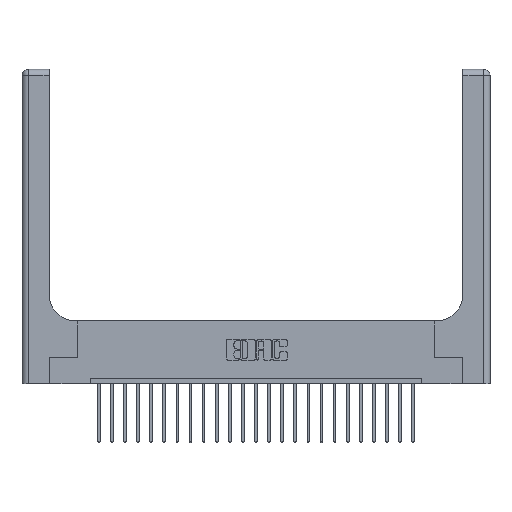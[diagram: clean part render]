
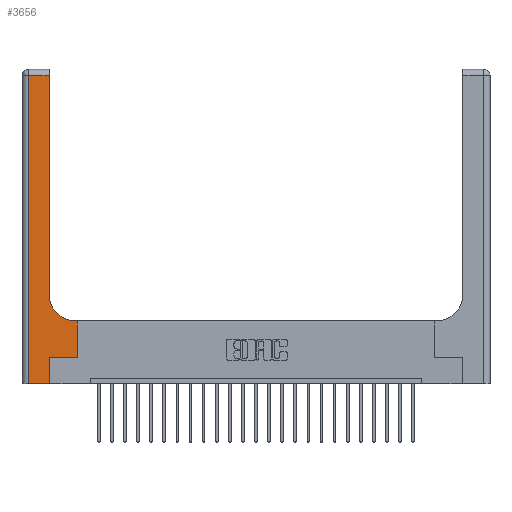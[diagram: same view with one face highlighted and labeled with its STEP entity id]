
A CAD part, top view. The second image highlights one B-rep face of the part: STEP entity #3656.
In plain terms, the highlighted planar face has unit normal (0, 0, 1).
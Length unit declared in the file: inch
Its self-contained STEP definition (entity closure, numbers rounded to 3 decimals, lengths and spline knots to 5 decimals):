
#551 = DIRECTION ( 'NONE',  ( 0., 0., -1. ) ) ;
#799 = VERTEX_POINT ( 'NONE', #23151 ) ;
#1366 = DIRECTION ( 'NONE',  ( 1., 0., 0. ) ) ;
#1512 = ORIENTED_EDGE ( 'NONE', *, *, #6271, .T. ) ;
#1781 = VERTEX_POINT ( 'NONE', #10018 ) ;
#2086 = CARTESIAN_POINT ( 'NONE',  ( 0., 3., 0.37 ) ) ;
#2209 = VECTOR ( 'NONE', #18904, 39.37008 ) ;
#2478 = DIRECTION ( 'NONE',  ( 0., 1., 0. ) ) ;
#2650 = DIRECTION ( 'NONE',  ( 0., 1., 0. ) ) ;
#2822 = CARTESIAN_POINT ( 'NONE',  ( 0.26, 3., 0.37 ) ) ;
#3233 = CARTESIAN_POINT ( 'NONE',  ( 0.528, 0.6, 0.37 ) ) ;
#3656 = ADVANCED_FACE ( 'NONE', ( #11100 ), #14774, .F. ) ;
#3767 = CARTESIAN_POINT ( 'NONE',  ( 0.51, 0.85, 0.37 ) ) ;
#4156 = EDGE_CURVE ( 'NONE', #10062, #5469, #22699, .T. ) ;
#4219 = ORIENTED_EDGE ( 'NONE', *, *, #8851, .T. ) ;
#4439 = CARTESIAN_POINT ( 'NONE',  ( 0.265, 0.25, 0.37 ) ) ;
#5050 = ORIENTED_EDGE ( 'NONE', *, *, #18211, .T. ) ;
#5339 = VECTOR ( 'NONE', #12613, 39.37008 ) ;
#5413 = DIRECTION ( 'NONE',  ( -1., 0., 0. ) ) ;
#5451 = DIRECTION ( 'NONE',  ( 0., 1., 0. ) ) ;
#5469 = VERTEX_POINT ( 'NONE', #4439 ) ;
#5524 = VERTEX_POINT ( 'NONE', #3233 ) ;
#5672 = DIRECTION ( 'NONE',  ( 1., 0., 0. ) ) ;
#6131 = ORIENTED_EDGE ( 'NONE', *, *, #11835, .T. ) ;
#6271 = EDGE_CURVE ( 'NONE', #17594, #15532, #16830, .T. ) ;
#7461 = LINE ( 'NONE', #18607, #12058 ) ;
#7475 = LINE ( 'NONE', #21704, #16451 ) ;
#7657 = ORIENTED_EDGE ( 'NONE', *, *, #4156, .T. ) ;
#7748 = VECTOR ( 'NONE', #2650, 39.37008 ) ;
#7778 = EDGE_CURVE ( 'NONE', #5469, #799, #18783, .T. ) ;
#8008 = CARTESIAN_POINT ( 'NONE',  ( 0.265, 0.25, 0.37 ) ) ;
#8629 = CARTESIAN_POINT ( 'NONE',  ( 0., 0., 0.37 ) ) ;
#8795 = VERTEX_POINT ( 'NONE', #20753 ) ;
#8851 = EDGE_CURVE ( 'NONE', #19646, #1781, #16408, .T. ) ;
#9235 = LINE ( 'NONE', #16573, #16431 ) ;
#10018 = CARTESIAN_POINT ( 'NONE',  ( 0.06, 0., 0.37 ) ) ;
#10062 = VERTEX_POINT ( 'NONE', #19322 ) ;
#10407 = AXIS2_PLACEMENT_3D ( 'NONE', #3767, #14675, #5672 ) ;
#11100 = FACE_OUTER_BOUND ( 'NONE', #19614, .T. ) ;
#11453 = ORIENTED_EDGE ( 'NONE', *, *, #18395, .T. ) ;
#11473 = ORIENTED_EDGE ( 'NONE', *, *, #7778, .T. ) ;
#11835 = EDGE_CURVE ( 'NONE', #15532, #19646, #9235, .T. ) ;
#11895 = CARTESIAN_POINT ( 'NONE',  ( 0.26, 0.85, 0.37 ) ) ;
#12058 = VECTOR ( 'NONE', #20272, 39.37008 ) ;
#12267 = LINE ( 'NONE', #8629, #23032 ) ;
#12419 = EDGE_CURVE ( 'NONE', #799, #5524, #7475, .T. ) ;
#12613 = DIRECTION ( 'NONE',  ( 0., -1., 0. ) ) ;
#12653 = CIRCLE ( 'NONE', #10407, 0.25 ) ;
#12757 = CARTESIAN_POINT ( 'NONE',  ( 0.26, 2.94, 0.37 ) ) ;
#13361 = ORIENTED_EDGE ( 'NONE', *, *, #12419, .T. ) ;
#13511 = ORIENTED_EDGE ( 'NONE', *, *, #14163, .T. ) ;
#14163 = EDGE_CURVE ( 'NONE', #8795, #17594, #12653, .T. ) ;
#14675 = DIRECTION ( 'NONE',  ( 0., 0., -1. ) ) ;
#14774 = PLANE ( 'NONE',  #14908 ) ;
#14908 = AXIS2_PLACEMENT_3D ( 'NONE', #2086, #551, #22260 ) ;
#15205 = CARTESIAN_POINT ( 'NONE',  ( 0.265, 0., 0.37 ) ) ;
#15532 = VERTEX_POINT ( 'NONE', #12757 ) ;
#16408 = LINE ( 'NONE', #21332, #5339 ) ;
#16431 = VECTOR ( 'NONE', #5413, 39.37008 ) ;
#16451 = VECTOR ( 'NONE', #5451, 39.37008 ) ;
#16573 = CARTESIAN_POINT ( 'NONE',  ( 0., 2.94, 0.37 ) ) ;
#16830 = LINE ( 'NONE', #2822, #18205 ) ;
#17594 = VERTEX_POINT ( 'NONE', #11895 ) ;
#18205 = VECTOR ( 'NONE', #2478, 39.37008 ) ;
#18211 = EDGE_CURVE ( 'NONE', #5524, #8795, #7461, .T. ) ;
#18395 = EDGE_CURVE ( 'NONE', #1781, #10062, #12267, .T. ) ;
#18607 = CARTESIAN_POINT ( 'NONE',  ( 0.26, 0.6, 0.37 ) ) ;
#18783 = LINE ( 'NONE', #8008, #2209 ) ;
#18904 = DIRECTION ( 'NONE',  ( 1., 0., 0. ) ) ;
#19322 = CARTESIAN_POINT ( 'NONE',  ( 0.265, 0., 0.37 ) ) ;
#19614 = EDGE_LOOP ( 'NONE', ( #1512, #6131, #4219, #11453, #7657, #11473, #13361, #5050, #13511 ) ) ;
#19646 = VERTEX_POINT ( 'NONE', #22285 ) ;
#20272 = DIRECTION ( 'NONE',  ( -1., 0., 0. ) ) ;
#20753 = CARTESIAN_POINT ( 'NONE',  ( 0.51, 0.6, 0.37 ) ) ;
#21332 = CARTESIAN_POINT ( 'NONE',  ( 0.06, 3., 0.37 ) ) ;
#21704 = CARTESIAN_POINT ( 'NONE',  ( 0.528, 0.25, 0.37 ) ) ;
#22260 = DIRECTION ( 'NONE',  ( -1., 0., 0. ) ) ;
#22285 = CARTESIAN_POINT ( 'NONE',  ( 0.06, 2.94, 0.37 ) ) ;
#22699 = LINE ( 'NONE', #15205, #7748 ) ;
#23032 = VECTOR ( 'NONE', #1366, 39.37008 ) ;
#23151 = CARTESIAN_POINT ( 'NONE',  ( 0.528, 0.25, 0.37 ) ) ;
